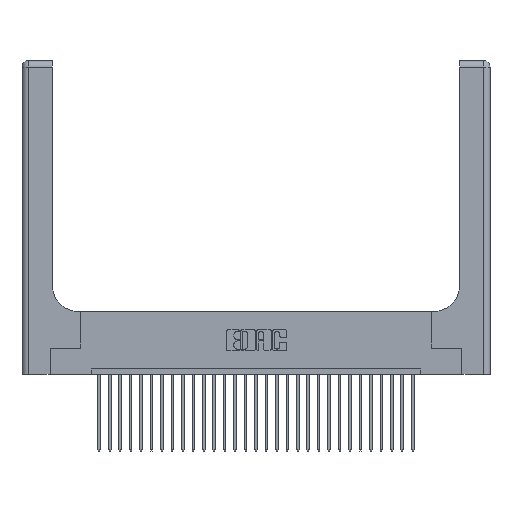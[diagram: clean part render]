
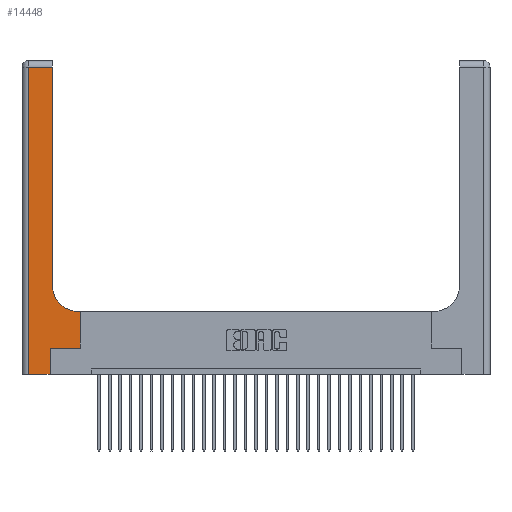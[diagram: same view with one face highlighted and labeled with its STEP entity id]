
A CAD part, top view. The second image highlights one B-rep face of the part: STEP entity #14448.
In plain terms, the highlighted planar face has unit normal (0, 0, 1).
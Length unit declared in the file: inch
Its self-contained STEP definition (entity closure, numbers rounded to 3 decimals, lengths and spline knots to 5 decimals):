
#25 = LINE ( 'NONE', #28927, #1488 ) ;
#348 = DIRECTION ( 'NONE',  ( 0., 0., -1. ) ) ;
#923 = EDGE_CURVE ( 'NONE', #23216, #3870, #23294, .T. ) ;
#1488 = VECTOR ( 'NONE', #5671, 39.37008 ) ;
#1597 = CARTESIAN_POINT ( 'NONE',  ( 0.5585, 0.6, 0.37 ) ) ;
#2513 = LINE ( 'NONE', #20266, #3241 ) ;
#2563 = DIRECTION ( 'NONE',  ( 1., 0., 0. ) ) ;
#3241 = VECTOR ( 'NONE', #4469, 39.37008 ) ;
#3804 = CARTESIAN_POINT ( 'NONE',  ( 0.5415, 0.6, 0.37 ) ) ;
#3870 = VERTEX_POINT ( 'NONE', #21391 ) ;
#4469 = DIRECTION ( 'NONE',  ( 1., 0., 0. ) ) ;
#4513 = DIRECTION ( 'NONE',  ( -1., 0., 0. ) ) ;
#5368 = DIRECTION ( 'NONE',  ( -1., 0., 0. ) ) ;
#5671 = DIRECTION ( 'NONE',  ( -1., 0., 0. ) ) ;
#5728 = EDGE_CURVE ( 'NONE', #9597, #8371, #10269, .T. ) ;
#6209 = DIRECTION ( 'NONE',  ( 1., 0., 0. ) ) ;
#6320 = VECTOR ( 'NONE', #12985, 39.37008 ) ;
#6430 = EDGE_CURVE ( 'NONE', #18350, #7146, #25, .T. ) ;
#6650 = CARTESIAN_POINT ( 'NONE',  ( 0.5585, 0.25, 0.37 ) ) ;
#7146 = VERTEX_POINT ( 'NONE', #3804 ) ;
#7866 = ORIENTED_EDGE ( 'NONE', *, *, #14202, .T. ) ;
#8020 = CARTESIAN_POINT ( 'NONE',  ( 0.06, 3., 0.37 ) ) ;
#8205 = ORIENTED_EDGE ( 'NONE', *, *, #5728, .T. ) ;
#8247 = CARTESIAN_POINT ( 'NONE',  ( 0.2915, 3., 0.37 ) ) ;
#8371 = VERTEX_POINT ( 'NONE', #6650 ) ;
#9220 = ORIENTED_EDGE ( 'NONE', *, *, #21276, .T. ) ;
#9597 = VERTEX_POINT ( 'NONE', #20147 ) ;
#10269 = LINE ( 'NONE', #18832, #24737 ) ;
#10665 = FACE_OUTER_BOUND ( 'NONE', #29342, .T. ) ;
#11262 = CARTESIAN_POINT ( 'NONE',  ( 0.5585, 0.25, 0.37 ) ) ;
#11976 = CARTESIAN_POINT ( 'NONE',  ( 0.2915, 2.94, 0.37 ) ) ;
#12038 = LINE ( 'NONE', #19391, #17441 ) ;
#12352 = CARTESIAN_POINT ( 'NONE',  ( 0., 2.94, 0.37 ) ) ;
#12985 = DIRECTION ( 'NONE',  ( 0., 1., 0. ) ) ;
#13078 = CARTESIAN_POINT ( 'NONE',  ( 0.269, 0., 0.37 ) ) ;
#13289 = VECTOR ( 'NONE', #26631, 39.37008 ) ;
#13382 = ORIENTED_EDGE ( 'NONE', *, *, #24516, .T. ) ;
#14202 = EDGE_CURVE ( 'NONE', #17368, #23216, #20796, .T. ) ;
#14448 = ADVANCED_FACE ( 'NONE', ( #10665 ), #18467, .F. ) ;
#15276 = EDGE_CURVE ( 'NONE', #26860, #9597, #12038, .T. ) ;
#15807 = CARTESIAN_POINT ( 'NONE',  ( 0.06, 0., 0.37 ) ) ;
#16178 = CARTESIAN_POINT ( 'NONE',  ( 0., 3., 0.37 ) ) ;
#16754 = VECTOR ( 'NONE', #5368, 39.37008 ) ;
#17368 = VERTEX_POINT ( 'NONE', #20790 ) ;
#17441 = VECTOR ( 'NONE', #21424, 39.37008 ) ;
#17528 = CARTESIAN_POINT ( 'NONE',  ( 0.5415, 0.85, 0.37 ) ) ;
#17802 = VERTEX_POINT ( 'NONE', #15807 ) ;
#18023 = DIRECTION ( 'NONE',  ( 0., 1., 0. ) ) ;
#18350 = VERTEX_POINT ( 'NONE', #1597 ) ;
#18359 = LINE ( 'NONE', #8020, #13289 ) ;
#18467 = PLANE ( 'NONE',  #21111 ) ;
#18481 = CIRCLE ( 'NONE', #21300, 0.25 ) ;
#18832 = CARTESIAN_POINT ( 'NONE',  ( 0.269, 0.25, 0.37 ) ) ;
#18895 = ORIENTED_EDGE ( 'NONE', *, *, #24650, .T. ) ;
#19316 = ORIENTED_EDGE ( 'NONE', *, *, #6430, .T. ) ;
#19391 = CARTESIAN_POINT ( 'NONE',  ( 0.269, 0., 0.37 ) ) ;
#20147 = CARTESIAN_POINT ( 'NONE',  ( 0.269, 0.25, 0.37 ) ) ;
#20266 = CARTESIAN_POINT ( 'NONE',  ( 0., 0., 0.37 ) ) ;
#20790 = CARTESIAN_POINT ( 'NONE',  ( 0.2915, 0.85, 0.37 ) ) ;
#20796 = LINE ( 'NONE', #8247, #6320 ) ;
#21018 = LINE ( 'NONE', #11262, #28298 ) ;
#21111 = AXIS2_PLACEMENT_3D ( 'NONE', #16178, #348, #4513 ) ;
#21276 = EDGE_CURVE ( 'NONE', #3870, #17802, #18359, .T. ) ;
#21300 = AXIS2_PLACEMENT_3D ( 'NONE', #17528, #22193, #6209 ) ;
#21391 = CARTESIAN_POINT ( 'NONE',  ( 0.06, 2.94, 0.37 ) ) ;
#21424 = DIRECTION ( 'NONE',  ( 0., 1., 0. ) ) ;
#22193 = DIRECTION ( 'NONE',  ( 0., 0., -1. ) ) ;
#23216 = VERTEX_POINT ( 'NONE', #11976 ) ;
#23253 = ORIENTED_EDGE ( 'NONE', *, *, #26365, .T. ) ;
#23294 = LINE ( 'NONE', #12352, #16754 ) ;
#24516 = EDGE_CURVE ( 'NONE', #7146, #17368, #18481, .T. ) ;
#24650 = EDGE_CURVE ( 'NONE', #8371, #18350, #21018, .T. ) ;
#24737 = VECTOR ( 'NONE', #2563, 39.37008 ) ;
#26365 = EDGE_CURVE ( 'NONE', #17802, #26860, #2513, .T. ) ;
#26631 = DIRECTION ( 'NONE',  ( 0., -1., 0. ) ) ;
#26860 = VERTEX_POINT ( 'NONE', #13078 ) ;
#28298 = VECTOR ( 'NONE', #18023, 39.37008 ) ;
#28497 = ORIENTED_EDGE ( 'NONE', *, *, #15276, .T. ) ;
#28927 = CARTESIAN_POINT ( 'NONE',  ( 0.2915, 0.6, 0.37 ) ) ;
#29342 = EDGE_LOOP ( 'NONE', ( #7866, #29619, #9220, #23253, #28497, #8205, #18895, #19316, #13382 ) ) ;
#29619 = ORIENTED_EDGE ( 'NONE', *, *, #923, .T. ) ;
